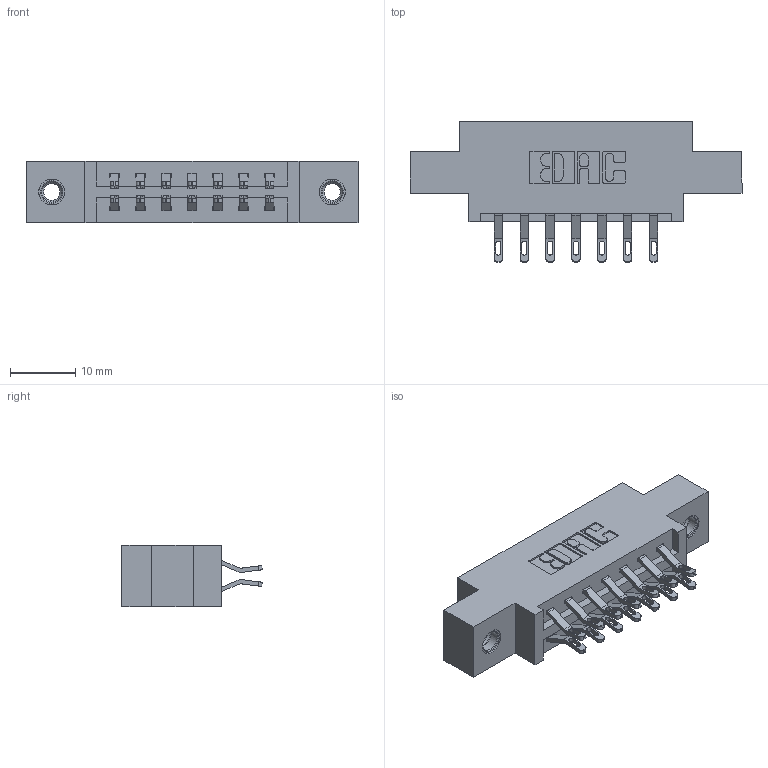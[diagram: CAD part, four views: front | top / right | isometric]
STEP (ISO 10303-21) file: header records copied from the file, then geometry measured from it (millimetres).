
FILE_DESCRIPTION (( 'STEP AP203' ), '1' );
FILE_NAME ('387-014-555-807.STEP', '2019-10-15T21:51:42', ( '' ), ( '' ), 'SwSTEP 2.0', 'SolidWorks 2016', '' );
FILE_SCHEMA (( 'CONFIG_CONTROL_DESIGN' ));
Length unit declared in the file: inch
Products named in the file (4): 345-250-001_345-250-005-103; 337 Part_0.170 Offset - 0.156 Dia-TI; 387-014-555-807; 345-292-001_555 Tail
Assembly tree (17 placements, depth 2):
  387-014-555-807
    337 Part_0.170 Offset - 0.156 Dia-TI
    345-292-001_555 Tail  x14
    345-250-001_345-250-005-103  x2
Bounding box: 50.75 x 21.47 x 9.4 mm (x, y, z)
Volume: 4792.1 mm3; surface area: 5374.3 mm2
Topology: 17 solids, 17 shells, 1018 faces, 3105 edges, 2062 vertices
Faces by surface type: plane 610, cylinder 392, cone 12, torus 4
Entity records: 11598 total; most frequent: CARTESIAN_POINT 1999, ORIENTED_EDGE 1898, DIRECTION 1767, EDGE_CURVE 949, VECTOR 781, LINE 781, VERTEX_POINT 628, AXIS2_PLACEMENT_3D 493
